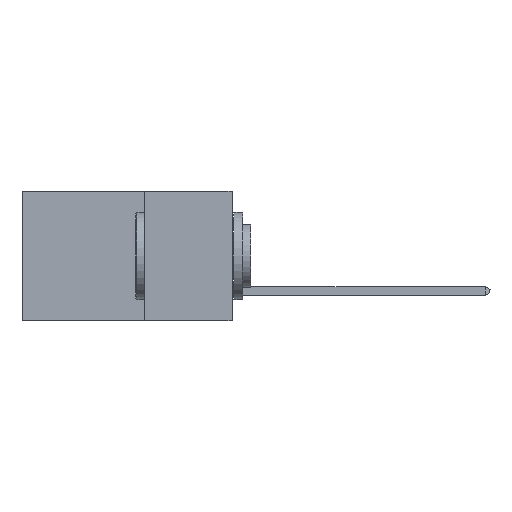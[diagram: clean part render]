
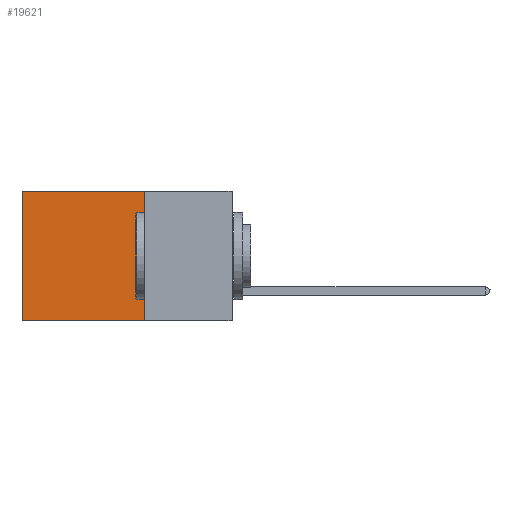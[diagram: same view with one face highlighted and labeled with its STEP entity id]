
A CAD part, left-side view. The second image highlights one B-rep face of the part: STEP entity #19621.
In plain terms, the highlighted planar face has unit normal (-1, 0, 0).
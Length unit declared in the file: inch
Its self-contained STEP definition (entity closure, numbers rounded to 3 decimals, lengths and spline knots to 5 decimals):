
#2049 = VERTEX_POINT ( 'NONE', #41022 ) ;
#3691 = CARTESIAN_POINT ( 'NONE',  ( 0.2875, 0.25, -0.37 ) ) ;
#5725 = ORIENTED_EDGE ( 'NONE', *, *, #39071, .F. ) ;
#6657 = VECTOR ( 'NONE', #16531, 39.37008 ) ;
#6673 = CARTESIAN_POINT ( 'NONE',  ( 0.2875, 0.25, 0. ) ) ;
#7193 = EDGE_CURVE ( 'NONE', #32116, #2049, #9885, .T. ) ;
#7683 = LINE ( 'NONE', #21476, #24169 ) ;
#9850 = CARTESIAN_POINT ( 'NONE',  ( 0.2875, 0.6, -0.37 ) ) ;
#9885 = LINE ( 'NONE', #33306, #39889 ) ;
#10166 = ORIENTED_EDGE ( 'NONE', *, *, #13226, .T. ) ;
#10964 = EDGE_CURVE ( 'NONE', #32116, #39920, #22373, .T. ) ;
#12385 = DIRECTION ( 'NONE',  ( 0., 0., -1. ) ) ;
#12729 = FACE_OUTER_BOUND ( 'NONE', #15280, .T. ) ;
#13226 = EDGE_CURVE ( 'NONE', #39920, #36033, #7683, .T. ) ;
#13227 = DIRECTION ( 'NONE',  ( 0., 0., -1. ) ) ;
#13387 = PLANE ( 'NONE',  #35402 ) ;
#14264 = ORIENTED_EDGE ( 'NONE', *, *, #7193, .F. ) ;
#14909 = VECTOR ( 'NONE', #30150, 39.37008 ) ;
#15280 = EDGE_LOOP ( 'NONE', ( #10166, #5725, #14264, #30263 ) ) ;
#16531 = DIRECTION ( 'NONE',  ( 0., 1., 0. ) ) ;
#19621 = ADVANCED_FACE ( 'NONE', ( #12729 ), #13387, .F. ) ;
#21476 = CARTESIAN_POINT ( 'NONE',  ( 0.2875, 0.6, 0. ) ) ;
#22373 = LINE ( 'NONE', #40101, #14909 ) ;
#24169 = VECTOR ( 'NONE', #12385, 39.37008 ) ;
#24982 = CARTESIAN_POINT ( 'NONE',  ( 0.2875, 0.25, 0. ) ) ;
#30150 = DIRECTION ( 'NONE',  ( 0., 1., 0. ) ) ;
#30263 = ORIENTED_EDGE ( 'NONE', *, *, #10964, .T. ) ;
#32116 = VERTEX_POINT ( 'NONE', #24982 ) ;
#33217 = CARTESIAN_POINT ( 'NONE',  ( 0.2875, 0.6, 0. ) ) ;
#33306 = CARTESIAN_POINT ( 'NONE',  ( 0.2875, 0.25, 0. ) ) ;
#35402 = AXIS2_PLACEMENT_3D ( 'NONE', #6673, #38656, #13227 ) ;
#36033 = VERTEX_POINT ( 'NONE', #9850 ) ;
#36099 = DIRECTION ( 'NONE',  ( 0., 0., -1. ) ) ;
#38656 = DIRECTION ( 'NONE',  ( 1., 0., 0. ) ) ;
#39071 = EDGE_CURVE ( 'NONE', #2049, #36033, #40692, .T. ) ;
#39889 = VECTOR ( 'NONE', #36099, 39.37008 ) ;
#39920 = VERTEX_POINT ( 'NONE', #33217 ) ;
#40101 = CARTESIAN_POINT ( 'NONE',  ( 0.2875, 0.25, 0. ) ) ;
#40692 = LINE ( 'NONE', #3691, #6657 ) ;
#41022 = CARTESIAN_POINT ( 'NONE',  ( 0.2875, 0.25, -0.37 ) ) ;
